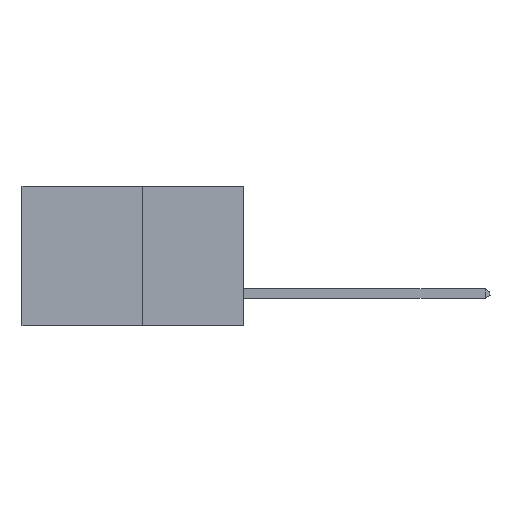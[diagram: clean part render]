
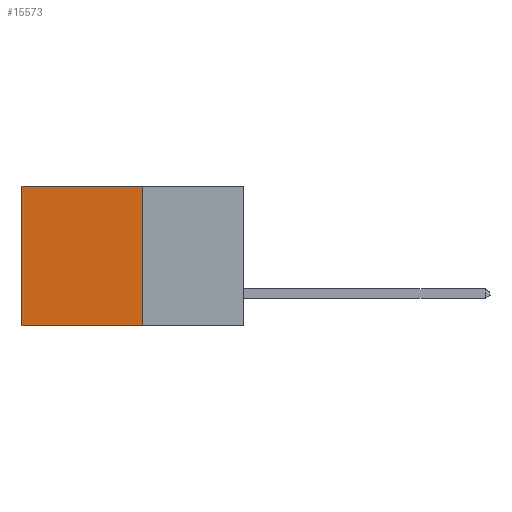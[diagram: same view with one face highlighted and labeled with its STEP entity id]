
A CAD part, left-side view. The second image highlights one B-rep face of the part: STEP entity #15573.
In plain terms, the highlighted planar face has unit normal (-1, 0, 0).
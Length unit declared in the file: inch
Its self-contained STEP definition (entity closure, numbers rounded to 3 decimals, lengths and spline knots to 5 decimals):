
#739 = EDGE_CURVE ( 'NONE', #32456, #11320, #30690, .T. ) ;
#954 = CARTESIAN_POINT ( 'NONE',  ( 0.277, 0.59, -0.37 ) ) ;
#1076 = DIRECTION ( 'NONE',  ( 0., 0., -1. ) ) ;
#4060 = VECTOR ( 'NONE', #1076, 39.37008 ) ;
#7113 = VECTOR ( 'NONE', #16895, 39.37008 ) ;
#7277 = PLANE ( 'NONE',  #7440 ) ;
#7386 = DIRECTION ( 'NONE',  ( 0., 1., 0. ) ) ;
#7440 = AXIS2_PLACEMENT_3D ( 'NONE', #24771, #9800, #27318 ) ;
#8434 = CARTESIAN_POINT ( 'NONE',  ( 0.277, 0.59, -0.37 ) ) ;
#9800 = DIRECTION ( 'NONE',  ( 1., 0., 0. ) ) ;
#10316 = EDGE_CURVE ( 'NONE', #20279, #11320, #19234, .T. ) ;
#10726 = CARTESIAN_POINT ( 'NONE',  ( 0.277, 0.27, -0.37 ) ) ;
#11320 = VERTEX_POINT ( 'NONE', #8434 ) ;
#11460 = CARTESIAN_POINT ( 'NONE',  ( 0.277, 0.27, -0.37 ) ) ;
#15573 = ADVANCED_FACE ( 'NONE', ( #25054 ), #7277, .F. ) ;
#16895 = DIRECTION ( 'NONE',  ( 0., 1., 0. ) ) ;
#17107 = CARTESIAN_POINT ( 'NONE',  ( 0.277, 0.59, 0. ) ) ;
#18081 = EDGE_CURVE ( 'NONE', #23139, #32456, #26305, .T. ) ;
#18194 = DIRECTION ( 'NONE',  ( 0., 0., -1. ) ) ;
#19234 = LINE ( 'NONE', #32323, #25852 ) ;
#20279 = VERTEX_POINT ( 'NONE', #11460 ) ;
#20590 = LINE ( 'NONE', #10726, #26413 ) ;
#21370 = ORIENTED_EDGE ( 'NONE', *, *, #739, .T. ) ;
#23139 = VERTEX_POINT ( 'NONE', #30101 ) ;
#24771 = CARTESIAN_POINT ( 'NONE',  ( 0.277, 0.27, -0.37 ) ) ;
#25054 = FACE_OUTER_BOUND ( 'NONE', #28205, .T. ) ;
#25852 = VECTOR ( 'NONE', #7386, 39.37008 ) ;
#26305 = LINE ( 'NONE', #31843, #7113 ) ;
#26413 = VECTOR ( 'NONE', #18194, 39.37008 ) ;
#26670 = ORIENTED_EDGE ( 'NONE', *, *, #10316, .F. ) ;
#27318 = DIRECTION ( 'NONE',  ( 0., 0., -1. ) ) ;
#28205 = EDGE_LOOP ( 'NONE', ( #21370, #26670, #28769, #29216 ) ) ;
#28769 = ORIENTED_EDGE ( 'NONE', *, *, #29145, .F. ) ;
#29145 = EDGE_CURVE ( 'NONE', #23139, #20279, #20590, .T. ) ;
#29216 = ORIENTED_EDGE ( 'NONE', *, *, #18081, .T. ) ;
#30101 = CARTESIAN_POINT ( 'NONE',  ( 0.277, 0.27, 0. ) ) ;
#30690 = LINE ( 'NONE', #954, #4060 ) ;
#31843 = CARTESIAN_POINT ( 'NONE',  ( 0.277, 0.27, 0. ) ) ;
#32323 = CARTESIAN_POINT ( 'NONE',  ( 0.277, 0.27, -0.37 ) ) ;
#32456 = VERTEX_POINT ( 'NONE', #17107 ) ;
